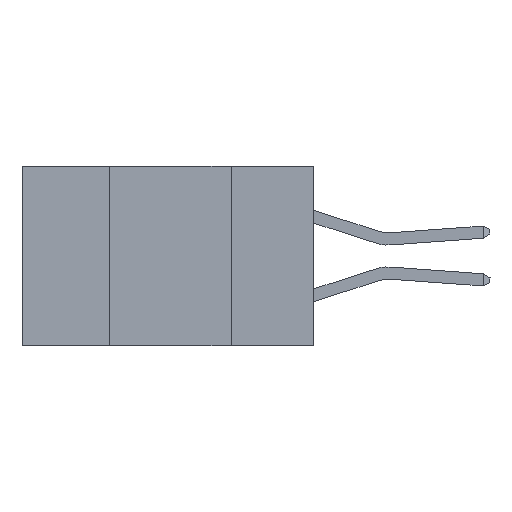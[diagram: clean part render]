
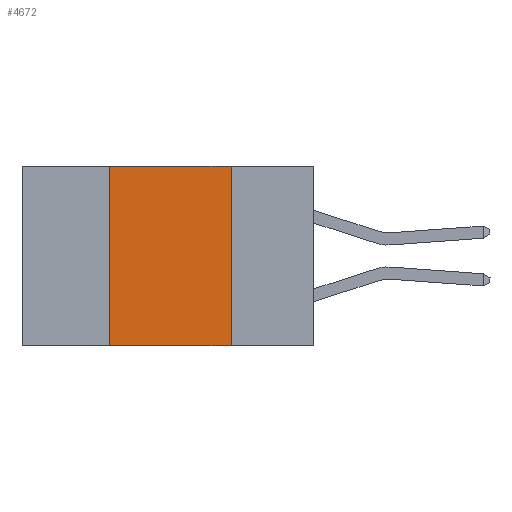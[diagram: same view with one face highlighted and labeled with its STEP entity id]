
A CAD part, left-side view. The second image highlights one B-rep face of the part: STEP entity #4672.
In plain terms, the highlighted planar face has unit normal (-1, 0, 0).
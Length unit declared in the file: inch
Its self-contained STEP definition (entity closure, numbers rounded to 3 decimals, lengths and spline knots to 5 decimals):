
#823 = ORIENTED_EDGE ( 'NONE', *, *, #4603, .F. ) ;
#984 = CARTESIAN_POINT ( 'NONE',  ( 0., 0.42, 0. ) ) ;
#988 = DIRECTION ( 'NONE',  ( 1., 0., 0. ) ) ;
#1102 = EDGE_CURVE ( 'NONE', #7555, #16849, #2559, .T. ) ;
#1370 = LINE ( 'NONE', #4446, #2140 ) ;
#2140 = VECTOR ( 'NONE', #15852, 39.37008 ) ;
#2559 = LINE ( 'NONE', #9923, #19172 ) ;
#3232 = DIRECTION ( 'NONE',  ( 0., -1., 0. ) ) ;
#4446 = CARTESIAN_POINT ( 'NONE',  ( 0., 0.17, 0. ) ) ;
#4603 = EDGE_CURVE ( 'NONE', #16849, #13971, #1370, .T. ) ;
#4672 = ADVANCED_FACE ( 'NONE', ( #18736 ), #18575, .F. ) ;
#5382 = EDGE_LOOP ( 'NONE', ( #823, #16941, #6527, #16871 ) ) ;
#5496 = CARTESIAN_POINT ( 'NONE',  ( 0., 0.17, 0. ) ) ;
#6503 = CARTESIAN_POINT ( 'NONE',  ( 0., 0.42, 0. ) ) ;
#6527 = ORIENTED_EDGE ( 'NONE', *, *, #6640, .F. ) ;
#6640 = EDGE_CURVE ( 'NONE', #13009, #7555, #13828, .T. ) ;
#7156 = DIRECTION ( 'NONE',  ( 0., -1., 0. ) ) ;
#7555 = VERTEX_POINT ( 'NONE', #984 ) ;
#9098 = CARTESIAN_POINT ( 'NONE',  ( 0., 0.6, 0. ) ) ;
#9923 = CARTESIAN_POINT ( 'NONE',  ( 0., 0.6, 0. ) ) ;
#9985 = LINE ( 'NONE', #13475, #10490 ) ;
#10490 = VECTOR ( 'NONE', #7156, 39.37008 ) ;
#10569 = DIRECTION ( 'NONE',  ( 0., 0., -1. ) ) ;
#10783 = CARTESIAN_POINT ( 'NONE',  ( 0., 0.42, -0.37 ) ) ;
#13009 = VERTEX_POINT ( 'NONE', #10783 ) ;
#13138 = DIRECTION ( 'NONE',  ( 0., 0., 1. ) ) ;
#13475 = CARTESIAN_POINT ( 'NONE',  ( 0., 0.6, -0.37 ) ) ;
#13828 = LINE ( 'NONE', #6503, #14355 ) ;
#13971 = VERTEX_POINT ( 'NONE', #17907 ) ;
#14355 = VECTOR ( 'NONE', #13138, 39.37008 ) ;
#15852 = DIRECTION ( 'NONE',  ( 0., 0., -1. ) ) ;
#15982 = AXIS2_PLACEMENT_3D ( 'NONE', #9098, #988, #10569 ) ;
#16849 = VERTEX_POINT ( 'NONE', #5496 ) ;
#16858 = EDGE_CURVE ( 'NONE', #13009, #13971, #9985, .T. ) ;
#16871 = ORIENTED_EDGE ( 'NONE', *, *, #16858, .T. ) ;
#16941 = ORIENTED_EDGE ( 'NONE', *, *, #1102, .F. ) ;
#17907 = CARTESIAN_POINT ( 'NONE',  ( 0., 0.17, -0.37 ) ) ;
#18575 = PLANE ( 'NONE',  #15982 ) ;
#18736 = FACE_OUTER_BOUND ( 'NONE', #5382, .T. ) ;
#19172 = VECTOR ( 'NONE', #3232, 39.37008 ) ;
